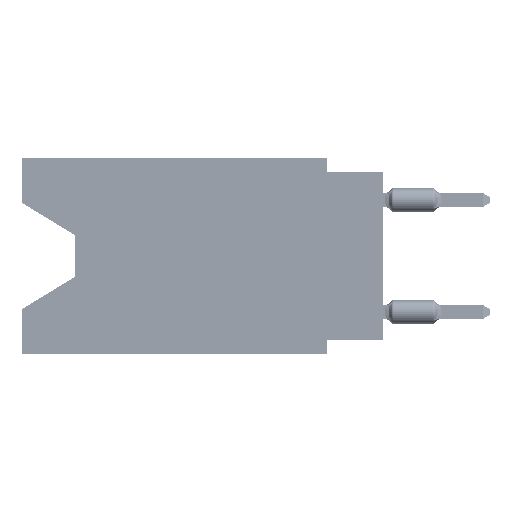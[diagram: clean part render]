
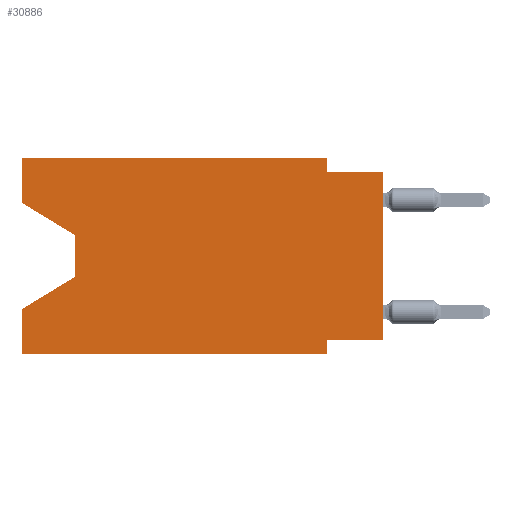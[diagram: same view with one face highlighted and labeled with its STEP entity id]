
A CAD part, left-side view. The second image highlights one B-rep face of the part: STEP entity #30886.
In plain terms, the highlighted planar face has unit normal (-1, 0, 0).
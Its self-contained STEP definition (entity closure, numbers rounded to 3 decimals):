
#39 = VECTOR ( 'NONE', #63754, 1000. ) ;
#1883 = CARTESIAN_POINT ( 'NONE',  ( 0., 0., -8.255 ) ) ;
#1940 = CARTESIAN_POINT ( 'NONE',  ( 0., 0., -8.255 ) ) ;
#5274 = CARTESIAN_POINT ( 'NONE',  ( 0., 16.383, -6.852 ) ) ;
#5326 = VECTOR ( 'NONE', #45983, 1000. ) ;
#5558 = VECTOR ( 'NONE', #47175, 1000. ) ;
#5729 = LINE ( 'NONE', #59121, #5326 ) ;
#6691 = CARTESIAN_POINT ( 'NONE',  ( 0., 16.383, -8.89 ) ) ;
#7369 = DIRECTION ( 'NONE',  ( 0., 0., -1. ) ) ;
#8327 = EDGE_CURVE ( 'NONE', #84502, #71570, #31792, .T. ) ;
#8807 = CARTESIAN_POINT ( 'NONE',  ( 0., 16.383, 0. ) ) ;
#9312 = EDGE_CURVE ( 'NONE', #30955, #52303, #17584, .T. ) ;
#11384 = VERTEX_POINT ( 'NONE', #32747 ) ;
#11418 = EDGE_CURVE ( 'NONE', #11384, #84502, #48032, .T. ) ;
#11858 = FACE_OUTER_BOUND ( 'NONE', #48635, .T. ) ;
#15590 = ORIENTED_EDGE ( 'NONE', *, *, #54396, .T. ) ;
#16483 = CARTESIAN_POINT ( 'NONE',  ( 0., 16.383, 0. ) ) ;
#16545 = LINE ( 'NONE', #62516, #53316 ) ;
#17584 = LINE ( 'NONE', #29838, #18344 ) ;
#17853 = LINE ( 'NONE', #44538, #72063 ) ;
#18293 = VECTOR ( 'NONE', #22134, 1000. ) ;
#18344 = VECTOR ( 'NONE', #77122, 1000. ) ;
#20494 = CARTESIAN_POINT ( 'NONE',  ( 0., 13.97, -5.385 ) ) ;
#20526 = CARTESIAN_POINT ( 'NONE',  ( 0., 16.383, -2.038 ) ) ;
#21715 = LINE ( 'NONE', #75101, #18293 ) ;
#22134 = DIRECTION ( 'NONE',  ( 0., -0.855, -0.519 ) ) ;
#22694 = DIRECTION ( 'NONE',  ( 0., -1., 0. ) ) ;
#22812 = VERTEX_POINT ( 'NONE', #16483 ) ;
#23168 = EDGE_CURVE ( 'NONE', #22812, #11384, #68386, .T. ) ;
#23457 = VERTEX_POINT ( 'NONE', #78424 ) ;
#26477 = CARTESIAN_POINT ( 'NONE',  ( 0., 2.54, -8.89 ) ) ;
#27733 = DIRECTION ( 'NONE',  ( 0., 1., 0. ) ) ;
#29348 = LINE ( 'NONE', #8807, #49907 ) ;
#29838 = CARTESIAN_POINT ( 'NONE',  ( 0., 2.54, -8.89 ) ) ;
#30110 = ORIENTED_EDGE ( 'NONE', *, *, #23168, .F. ) ;
#30886 = ADVANCED_FACE ( 'NONE', ( #11858 ), #79691, .F. ) ;
#30955 = VERTEX_POINT ( 'NONE', #47259 ) ;
#31792 = LINE ( 'NONE', #57618, #39 ) ;
#32747 = CARTESIAN_POINT ( 'NONE',  ( 0., 2.54, 0. ) ) ;
#32817 = VERTEX_POINT ( 'NONE', #5274 ) ;
#34235 = AXIS2_PLACEMENT_3D ( 'NONE', #58251, #46389, #73117 ) ;
#35281 = ORIENTED_EDGE ( 'NONE', *, *, #56617, .T. ) ;
#35409 = VERTEX_POINT ( 'NONE', #6691 ) ;
#35572 = LINE ( 'NONE', #1883, #39744 ) ;
#36022 = ORIENTED_EDGE ( 'NONE', *, *, #71006, .T. ) ;
#37342 = ORIENTED_EDGE ( 'NONE', *, *, #42895, .T. ) ;
#38193 = EDGE_CURVE ( 'NONE', #35409, #32817, #29348, .T. ) ;
#39307 = CARTESIAN_POINT ( 'NONE',  ( 0., 2.54, -0.635 ) ) ;
#39744 = VECTOR ( 'NONE', #27733, 1000. ) ;
#41026 = ORIENTED_EDGE ( 'NONE', *, *, #51719, .F. ) ;
#42895 = EDGE_CURVE ( 'NONE', #44667, #52285, #21715, .T. ) ;
#44538 = CARTESIAN_POINT ( 'NONE',  ( 0., 16.383, 0. ) ) ;
#44667 = VERTEX_POINT ( 'NONE', #20526 ) ;
#45710 = ORIENTED_EDGE ( 'NONE', *, *, #11418, .F. ) ;
#45983 = DIRECTION ( 'NONE',  ( 0., 0., -1. ) ) ;
#46389 = DIRECTION ( 'NONE',  ( 1., 0., 0. ) ) ;
#47175 = DIRECTION ( 'NONE',  ( 0., 0.855, -0.519 ) ) ;
#47259 = CARTESIAN_POINT ( 'NONE',  ( 0., 2.54, -8.255 ) ) ;
#48032 = LINE ( 'NONE', #67318, #81601 ) ;
#48635 = EDGE_LOOP ( 'NONE', ( #37342, #15590, #35281, #82418, #36022, #65355, #70185, #74059, #57487, #45710, #30110, #41026 ) ) ;
#49907 = VECTOR ( 'NONE', #83185, 1000. ) ;
#51719 = EDGE_CURVE ( 'NONE', #44667, #22812, #17853, .T. ) ;
#52285 = VERTEX_POINT ( 'NONE', #59753 ) ;
#52303 = VERTEX_POINT ( 'NONE', #26477 ) ;
#52422 = DIRECTION ( 'NONE',  ( 0., 0., 1. ) ) ;
#53316 = VECTOR ( 'NONE', #22694, 1000. ) ;
#53954 = CARTESIAN_POINT ( 'NONE',  ( 0., 16.383, 0. ) ) ;
#54396 = EDGE_CURVE ( 'NONE', #52285, #23457, #5729, .T. ) ;
#55697 = VECTOR ( 'NONE', #64260, 1000. ) ;
#56617 = EDGE_CURVE ( 'NONE', #23457, #32817, #80893, .T. ) ;
#56993 = VECTOR ( 'NONE', #74099, 1000. ) ;
#57487 = ORIENTED_EDGE ( 'NONE', *, *, #8327, .F. ) ;
#57618 = CARTESIAN_POINT ( 'NONE',  ( 0., 0., -0.635 ) ) ;
#58251 = CARTESIAN_POINT ( 'NONE',  ( 0., 16.383, 0. ) ) ;
#58774 = CARTESIAN_POINT ( 'NONE',  ( 0., 0., -0.635 ) ) ;
#59121 = CARTESIAN_POINT ( 'NONE',  ( 0., 13.97, -3.505 ) ) ;
#59753 = CARTESIAN_POINT ( 'NONE',  ( 0., 13.97, -3.505 ) ) ;
#62516 = CARTESIAN_POINT ( 'NONE',  ( 0., 16.383, -8.89 ) ) ;
#63754 = DIRECTION ( 'NONE',  ( 0., -1., 0. ) ) ;
#64260 = DIRECTION ( 'NONE',  ( 0., 0., 1. ) ) ;
#65355 = ORIENTED_EDGE ( 'NONE', *, *, #9312, .F. ) ;
#65513 = EDGE_CURVE ( 'NONE', #68276, #71570, #78715, .T. ) ;
#67318 = CARTESIAN_POINT ( 'NONE',  ( 0., 2.54, 0. ) ) ;
#68276 = VERTEX_POINT ( 'NONE', #1940 ) ;
#68386 = LINE ( 'NONE', #53954, #56993 ) ;
#70185 = ORIENTED_EDGE ( 'NONE', *, *, #75617, .F. ) ;
#71006 = EDGE_CURVE ( 'NONE', #35409, #52303, #16545, .T. ) ;
#71570 = VERTEX_POINT ( 'NONE', #58774 ) ;
#72063 = VECTOR ( 'NONE', #52422, 1000. ) ;
#73117 = DIRECTION ( 'NONE',  ( 0., 0., -1. ) ) ;
#74059 = ORIENTED_EDGE ( 'NONE', *, *, #65513, .T. ) ;
#74099 = DIRECTION ( 'NONE',  ( 0., -1., 0. ) ) ;
#75101 = CARTESIAN_POINT ( 'NONE',  ( 0., 16.383, -2.038 ) ) ;
#75617 = EDGE_CURVE ( 'NONE', #68276, #30955, #35572, .T. ) ;
#76969 = CARTESIAN_POINT ( 'NONE',  ( 0., 0., 0. ) ) ;
#77122 = DIRECTION ( 'NONE',  ( 0., 0., -1. ) ) ;
#78424 = CARTESIAN_POINT ( 'NONE',  ( 0., 13.97, -5.385 ) ) ;
#78715 = LINE ( 'NONE', #76969, #55697 ) ;
#79691 = PLANE ( 'NONE',  #34235 ) ;
#80893 = LINE ( 'NONE', #20494, #5558 ) ;
#81601 = VECTOR ( 'NONE', #7369, 1000. ) ;
#82418 = ORIENTED_EDGE ( 'NONE', *, *, #38193, .F. ) ;
#83185 = DIRECTION ( 'NONE',  ( 0., 0., 1. ) ) ;
#84502 = VERTEX_POINT ( 'NONE', #39307 ) ;
